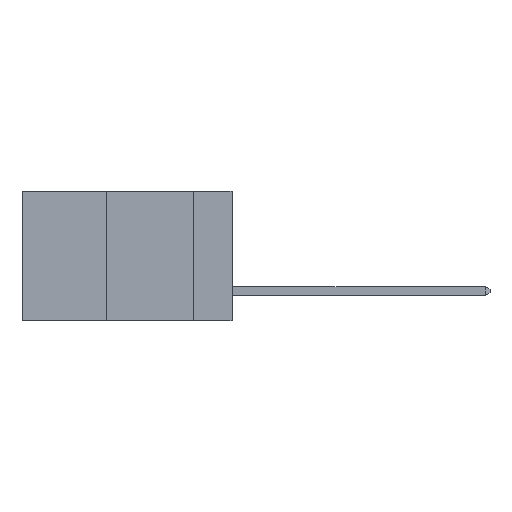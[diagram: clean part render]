
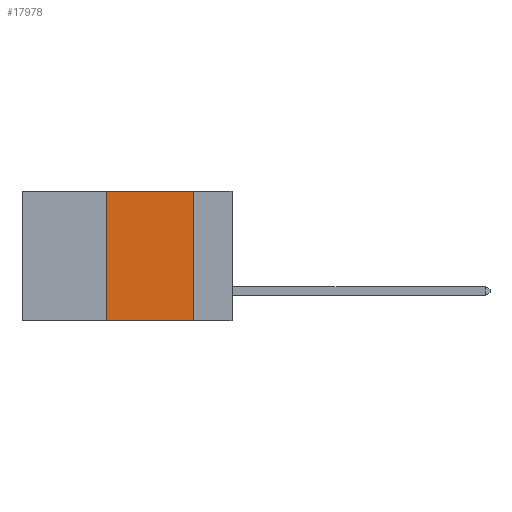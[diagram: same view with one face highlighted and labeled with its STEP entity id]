
A CAD part, left-side view. The second image highlights one B-rep face of the part: STEP entity #17978.
In plain terms, the highlighted planar face has unit normal (-1, 0, 0).
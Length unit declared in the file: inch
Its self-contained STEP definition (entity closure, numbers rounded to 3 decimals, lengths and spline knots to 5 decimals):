
#438 = LINE ( 'NONE', #11707, #16411 ) ;
#941 = VERTEX_POINT ( 'NONE', #3389 ) ;
#1176 = PLANE ( 'NONE',  #9458 ) ;
#2025 = LINE ( 'NONE', #13992, #17071 ) ;
#3389 = CARTESIAN_POINT ( 'NONE',  ( 0., 0.11, 0. ) ) ;
#4242 = VECTOR ( 'NONE', #18296, 39.37008 ) ;
#4505 = FACE_OUTER_BOUND ( 'NONE', #24565, .T. ) ;
#6318 = CARTESIAN_POINT ( 'NONE',  ( 0., 0.11, -0.37 ) ) ;
#6612 = EDGE_CURVE ( 'NONE', #14559, #941, #27251, .T. ) ;
#7242 = DIRECTION ( 'NONE',  ( 0., 0., -1. ) ) ;
#7645 = VERTEX_POINT ( 'NONE', #20112 ) ;
#7973 = DIRECTION ( 'NONE',  ( 0., 0., 1. ) ) ;
#9458 = AXIS2_PLACEMENT_3D ( 'NONE', #22192, #25228, #7242 ) ;
#9542 = DIRECTION ( 'NONE',  ( 0., -1., 0. ) ) ;
#9826 = VERTEX_POINT ( 'NONE', #6318 ) ;
#11265 = LINE ( 'NONE', #36279, #4242 ) ;
#11603 = EDGE_CURVE ( 'NONE', #7645, #9826, #11265, .T. ) ;
#11707 = CARTESIAN_POINT ( 'NONE',  ( 0., 0.11, 0. ) ) ;
#13992 = CARTESIAN_POINT ( 'NONE',  ( 0., 0.36, 0. ) ) ;
#14559 = VERTEX_POINT ( 'NONE', #35057 ) ;
#16411 = VECTOR ( 'NONE', #17775, 39.37008 ) ;
#16542 = ORIENTED_EDGE ( 'NONE', *, *, #30537, .F. ) ;
#17071 = VECTOR ( 'NONE', #7973, 39.37008 ) ;
#17775 = DIRECTION ( 'NONE',  ( 0., 0., -1. ) ) ;
#17978 = ADVANCED_FACE ( 'NONE', ( #4505 ), #1176, .F. ) ;
#18296 = DIRECTION ( 'NONE',  ( 0., -1., 0. ) ) ;
#19261 = VECTOR ( 'NONE', #9542, 39.37008 ) ;
#20112 = CARTESIAN_POINT ( 'NONE',  ( 0., 0.36, -0.37 ) ) ;
#21690 = EDGE_CURVE ( 'NONE', #941, #9826, #438, .T. ) ;
#22192 = CARTESIAN_POINT ( 'NONE',  ( 0., 0.6, 0. ) ) ;
#24487 = CARTESIAN_POINT ( 'NONE',  ( 0., 0.6, 0. ) ) ;
#24565 = EDGE_LOOP ( 'NONE', ( #33535, #26008, #16542, #24781 ) ) ;
#24781 = ORIENTED_EDGE ( 'NONE', *, *, #11603, .T. ) ;
#25228 = DIRECTION ( 'NONE',  ( 1., 0., 0. ) ) ;
#26008 = ORIENTED_EDGE ( 'NONE', *, *, #6612, .F. ) ;
#27251 = LINE ( 'NONE', #24487, #19261 ) ;
#30537 = EDGE_CURVE ( 'NONE', #7645, #14559, #2025, .T. ) ;
#33535 = ORIENTED_EDGE ( 'NONE', *, *, #21690, .F. ) ;
#35057 = CARTESIAN_POINT ( 'NONE',  ( 0., 0.36, 0. ) ) ;
#36279 = CARTESIAN_POINT ( 'NONE',  ( 0., 0.6, -0.37 ) ) ;
